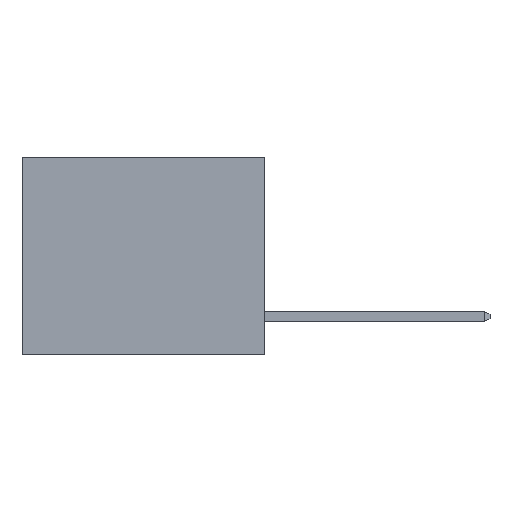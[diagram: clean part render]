
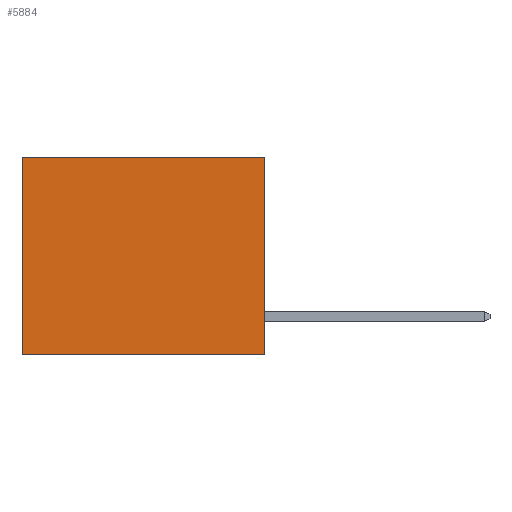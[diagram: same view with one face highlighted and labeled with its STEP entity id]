
A CAD part, left-side view. The second image highlights one B-rep face of the part: STEP entity #5884.
In plain terms, the highlighted planar face has unit normal (-1, 0, 0).
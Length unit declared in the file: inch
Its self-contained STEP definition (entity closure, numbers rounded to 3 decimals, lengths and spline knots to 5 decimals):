
#25 = CARTESIAN_POINT ( 'NONE',  ( 0.3165, 0., -0.49 ) ) ;
#469 = DIRECTION ( 'NONE',  ( 0., 1., 0. ) ) ;
#658 = VERTEX_POINT ( 'NONE', #3522 ) ;
#898 = VECTOR ( 'NONE', #5810, 39.37008 ) ;
#1147 = LINE ( 'NONE', #3702, #4906 ) ;
#1166 = ORIENTED_EDGE ( 'NONE', *, *, #3193, .T. ) ;
#1254 = ORIENTED_EDGE ( 'NONE', *, *, #1589, .F. ) ;
#1310 = CARTESIAN_POINT ( 'NONE',  ( 0.3165, 0.6, -0.49 ) ) ;
#1357 = CARTESIAN_POINT ( 'NONE',  ( 0.3165, 0.6, 0. ) ) ;
#1510 = CARTESIAN_POINT ( 'NONE',  ( 0.3165, 0., -0.49 ) ) ;
#1589 = EDGE_CURVE ( 'NONE', #658, #4967, #6123, .T. ) ;
#1667 = CARTESIAN_POINT ( 'NONE',  ( 0.3165, 0.6, -0.49 ) ) ;
#1892 = LINE ( 'NONE', #4771, #6931 ) ;
#2126 = CARTESIAN_POINT ( 'NONE',  ( 0.3165, 0., -0.49 ) ) ;
#2138 = ORIENTED_EDGE ( 'NONE', *, *, #6087, .F. ) ;
#2400 = EDGE_LOOP ( 'NONE', ( #1166, #2138, #1254, #7125 ) ) ;
#2926 = LINE ( 'NONE', #1310, #6699 ) ;
#3193 = EDGE_CURVE ( 'NONE', #5072, #4290, #2926, .T. ) ;
#3522 = CARTESIAN_POINT ( 'NONE',  ( 0.3165, 0., 0. ) ) ;
#3702 = CARTESIAN_POINT ( 'NONE',  ( 0.3165, 0., -0.49 ) ) ;
#4159 = AXIS2_PLACEMENT_3D ( 'NONE', #1510, #5173, #5251 ) ;
#4290 = VERTEX_POINT ( 'NONE', #1667 ) ;
#4771 = CARTESIAN_POINT ( 'NONE',  ( 0.3165, 0., 0. ) ) ;
#4906 = VECTOR ( 'NONE', #6119, 39.37008 ) ;
#4967 = VERTEX_POINT ( 'NONE', #25 ) ;
#5072 = VERTEX_POINT ( 'NONE', #1357 ) ;
#5173 = DIRECTION ( 'NONE',  ( 1., 0., 0. ) ) ;
#5251 = DIRECTION ( 'NONE',  ( 0., 0., -1. ) ) ;
#5810 = DIRECTION ( 'NONE',  ( 0., 0., -1. ) ) ;
#5884 = ADVANCED_FACE ( 'NONE', ( #6768 ), #7788, .F. ) ;
#6087 = EDGE_CURVE ( 'NONE', #4967, #4290, #1147, .T. ) ;
#6119 = DIRECTION ( 'NONE',  ( 0., 1., 0. ) ) ;
#6123 = LINE ( 'NONE', #2126, #898 ) ;
#6278 = DIRECTION ( 'NONE',  ( 0., 0., -1. ) ) ;
#6699 = VECTOR ( 'NONE', #6278, 39.37008 ) ;
#6768 = FACE_OUTER_BOUND ( 'NONE', #2400, .T. ) ;
#6928 = EDGE_CURVE ( 'NONE', #658, #5072, #1892, .T. ) ;
#6931 = VECTOR ( 'NONE', #469, 39.37008 ) ;
#7125 = ORIENTED_EDGE ( 'NONE', *, *, #6928, .T. ) ;
#7788 = PLANE ( 'NONE',  #4159 ) ;
